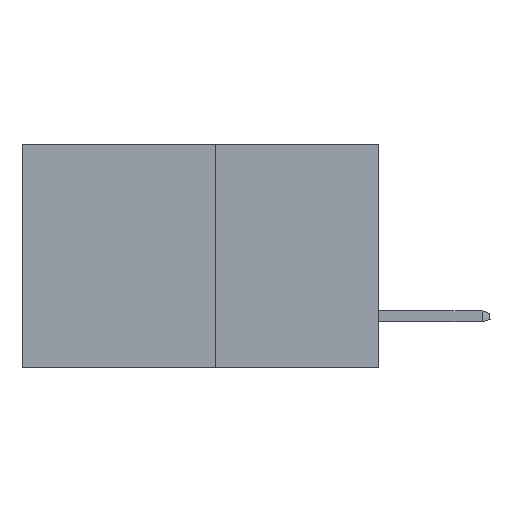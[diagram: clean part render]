
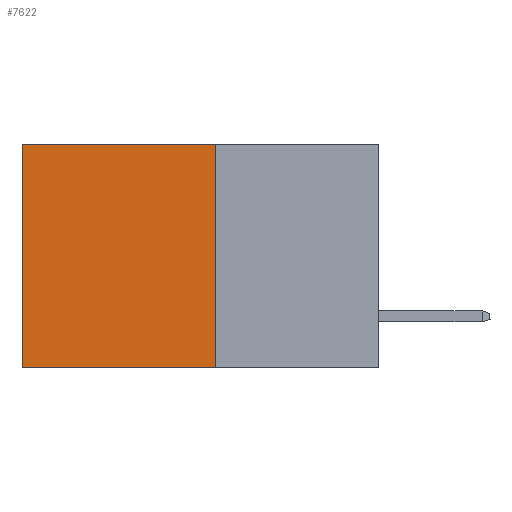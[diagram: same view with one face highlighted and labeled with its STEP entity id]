
A CAD part, left-side view. The second image highlights one B-rep face of the part: STEP entity #7622.
In plain terms, the highlighted planar face has unit normal (-1, 0, 0).
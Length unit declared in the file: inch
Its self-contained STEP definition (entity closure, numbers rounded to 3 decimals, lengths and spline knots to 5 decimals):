
#54 = DIRECTION ( 'NONE',  ( 0., 1., 0. ) ) ;
#1146 = VERTEX_POINT ( 'NONE', #8403 ) ;
#1206 = ORIENTED_EDGE ( 'NONE', *, *, #9170, .T. ) ;
#1332 = CARTESIAN_POINT ( 'NONE',  ( 0.277, 0.27, 0. ) ) ;
#1400 = VERTEX_POINT ( 'NONE', #2749 ) ;
#1546 = CARTESIAN_POINT ( 'NONE',  ( 0.277, 0.27, -0.37 ) ) ;
#1607 = DIRECTION ( 'NONE',  ( 0., 0., -1. ) ) ;
#1750 = LINE ( 'NONE', #1332, #8409 ) ;
#1753 = FACE_OUTER_BOUND ( 'NONE', #8341, .T. ) ;
#2745 = LINE ( 'NONE', #17410, #16636 ) ;
#2749 = CARTESIAN_POINT ( 'NONE',  ( 0.277, 0.27, 0. ) ) ;
#3013 = ORIENTED_EDGE ( 'NONE', *, *, #11680, .F. ) ;
#3465 = VECTOR ( 'NONE', #6458, 39.37008 ) ;
#4388 = VERTEX_POINT ( 'NONE', #15094 ) ;
#4740 = AXIS2_PLACEMENT_3D ( 'NONE', #1546, #9996, #1607 ) ;
#6458 = DIRECTION ( 'NONE',  ( 0., 0., -1. ) ) ;
#7622 = ADVANCED_FACE ( 'NONE', ( #1753 ), #8672, .F. ) ;
#8225 = EDGE_CURVE ( 'NONE', #1146, #4388, #9834, .T. ) ;
#8341 = EDGE_LOOP ( 'NONE', ( #1206, #13028, #3013, #9006 ) ) ;
#8403 = CARTESIAN_POINT ( 'NONE',  ( 0.277, 0.27, -0.37 ) ) ;
#8409 = VECTOR ( 'NONE', #9674, 39.37008 ) ;
#8672 = PLANE ( 'NONE',  #4740 ) ;
#9006 = ORIENTED_EDGE ( 'NONE', *, *, #16953, .T. ) ;
#9170 = EDGE_CURVE ( 'NONE', #13804, #4388, #2745, .T. ) ;
#9427 = VECTOR ( 'NONE', #54, 39.37008 ) ;
#9674 = DIRECTION ( 'NONE',  ( 0., 1., 0. ) ) ;
#9834 = LINE ( 'NONE', #11227, #9427 ) ;
#9996 = DIRECTION ( 'NONE',  ( 1., 0., 0. ) ) ;
#10604 = DIRECTION ( 'NONE',  ( 0., 0., -1. ) ) ;
#11227 = CARTESIAN_POINT ( 'NONE',  ( 0.277, 0.27, -0.37 ) ) ;
#11680 = EDGE_CURVE ( 'NONE', #1400, #1146, #11752, .T. ) ;
#11752 = LINE ( 'NONE', #15987, #3465 ) ;
#13028 = ORIENTED_EDGE ( 'NONE', *, *, #8225, .F. ) ;
#13804 = VERTEX_POINT ( 'NONE', #14217 ) ;
#14217 = CARTESIAN_POINT ( 'NONE',  ( 0.277, 0.59, 0. ) ) ;
#15094 = CARTESIAN_POINT ( 'NONE',  ( 0.277, 0.59, -0.37 ) ) ;
#15987 = CARTESIAN_POINT ( 'NONE',  ( 0.277, 0.27, -0.37 ) ) ;
#16636 = VECTOR ( 'NONE', #10604, 39.37008 ) ;
#16953 = EDGE_CURVE ( 'NONE', #1400, #13804, #1750, .T. ) ;
#17410 = CARTESIAN_POINT ( 'NONE',  ( 0.277, 0.59, -0.37 ) ) ;
